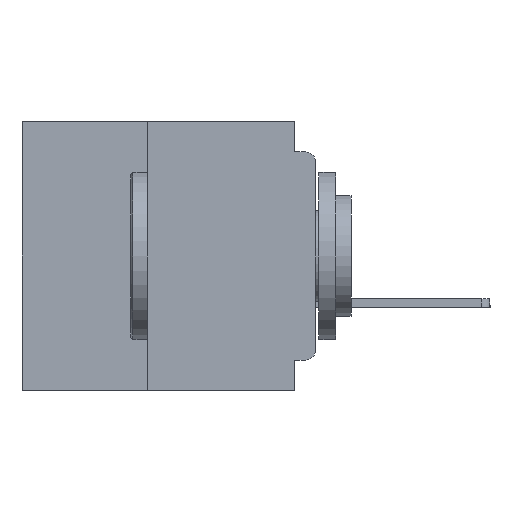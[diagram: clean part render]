
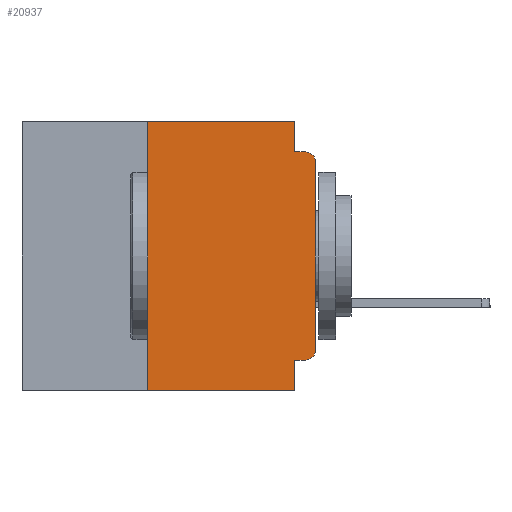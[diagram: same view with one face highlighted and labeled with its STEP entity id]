
A CAD part, left-side view. The second image highlights one B-rep face of the part: STEP entity #20937.
In plain terms, the highlighted planar face has unit normal (-1, 0, 0).
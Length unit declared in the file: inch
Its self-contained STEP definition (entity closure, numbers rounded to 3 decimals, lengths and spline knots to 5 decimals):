
#1321 = LINE ( 'NONE', #22368, #30755 ) ;
#1678 = CARTESIAN_POINT ( 'NONE',  ( 0., 0.25, -0.4 ) ) ;
#2485 = DIRECTION ( 'NONE',  ( 0., 0., -1. ) ) ;
#2578 = VERTEX_POINT ( 'NONE', #18800 ) ;
#4115 = VERTEX_POINT ( 'NONE', #20687 ) ;
#4446 = CARTESIAN_POINT ( 'NONE',  ( 0., 0.031, 0. ) ) ;
#5508 = EDGE_CURVE ( 'NONE', #21175, #4115, #17553, .T. ) ;
#6006 = PLANE ( 'NONE',  #22523 ) ;
#6417 = FACE_OUTER_BOUND ( 'NONE', #26685, .T. ) ;
#6461 = CARTESIAN_POINT ( 'NONE',  ( 0., 0., -0.34 ) ) ;
#6690 = ORIENTED_EDGE ( 'NONE', *, *, #34855, .F. ) ;
#6709 = VECTOR ( 'NONE', #27355, 39.37008 ) ;
#6992 = CIRCLE ( 'NONE', #20363, 0.015 ) ;
#7013 = DIRECTION ( 'NONE',  ( 0., 1., 0. ) ) ;
#7372 = CARTESIAN_POINT ( 'NONE',  ( 0., 0.015, -0.06 ) ) ;
#7402 = EDGE_CURVE ( 'NONE', #34662, #21175, #11601, .T. ) ;
#8612 = VERTEX_POINT ( 'NONE', #4446 ) ;
#8872 = DIRECTION ( 'NONE',  ( 0., 0., -1. ) ) ;
#9820 = CARTESIAN_POINT ( 'NONE',  ( 0., 0.437, -0.4 ) ) ;
#10241 = DIRECTION ( 'NONE',  ( 0., 0., -1. ) ) ;
#10256 = VECTOR ( 'NONE', #13206, 39.37008 ) ;
#10634 = VECTOR ( 'NONE', #2485, 39.37008 ) ;
#10846 = VERTEX_POINT ( 'NONE', #33347 ) ;
#10946 = CARTESIAN_POINT ( 'NONE',  ( 0., 0., -0.045 ) ) ;
#11540 = LINE ( 'NONE', #30866, #10634 ) ;
#11601 = LINE ( 'NONE', #24078, #19231 ) ;
#12197 = CARTESIAN_POINT ( 'NONE',  ( 0., 0.015, -0.355 ) ) ;
#13206 = DIRECTION ( 'NONE',  ( 0., -1., 0. ) ) ;
#13582 = VERTEX_POINT ( 'NONE', #17877 ) ;
#13806 = DIRECTION ( 'NONE',  ( 0., 0., 1. ) ) ;
#13849 = DIRECTION ( 'NONE',  ( 0., -1., 0. ) ) ;
#14216 = ORIENTED_EDGE ( 'NONE', *, *, #5508, .F. ) ;
#14346 = LINE ( 'NONE', #1678, #6709 ) ;
#14812 = ORIENTED_EDGE ( 'NONE', *, *, #19490, .T. ) ;
#15301 = CIRCLE ( 'NONE', #19650, 0.015 ) ;
#16126 = CARTESIAN_POINT ( 'NONE',  ( 0., 0.015, -0.34 ) ) ;
#16238 = ORIENTED_EDGE ( 'NONE', *, *, #29856, .F. ) ;
#16655 = VECTOR ( 'NONE', #26226, 39.37008 ) ;
#17297 = ORIENTED_EDGE ( 'NONE', *, *, #30413, .T. ) ;
#17553 = LINE ( 'NONE', #31826, #16655 ) ;
#17877 = CARTESIAN_POINT ( 'NONE',  ( 0., 0.015, -0.045 ) ) ;
#18475 = DIRECTION ( 'NONE',  ( 0., -1., 0. ) ) ;
#18492 = EDGE_CURVE ( 'NONE', #8612, #2578, #11540, .T. ) ;
#18631 = CARTESIAN_POINT ( 'NONE',  ( 0., 0.031, -0.355 ) ) ;
#18800 = CARTESIAN_POINT ( 'NONE',  ( 0., 0.031, -0.045 ) ) ;
#18992 = DIRECTION ( 'NONE',  ( 0., 0., -1. ) ) ;
#19231 = VECTOR ( 'NONE', #7013, 39.37008 ) ;
#19295 = ORIENTED_EDGE ( 'NONE', *, *, #28532, .T. ) ;
#19490 = EDGE_CURVE ( 'NONE', #34662, #29398, #6992, .T. ) ;
#19650 = AXIS2_PLACEMENT_3D ( 'NONE', #7372, #27225, #10241 ) ;
#20363 = AXIS2_PLACEMENT_3D ( 'NONE', #16126, #35873, #18992 ) ;
#20687 = CARTESIAN_POINT ( 'NONE',  ( 0., 0.031, -0.4 ) ) ;
#20937 = ADVANCED_FACE ( 'NONE', ( #6417 ), #6006, .F. ) ;
#21175 = VERTEX_POINT ( 'NONE', #18631 ) ;
#21303 = VERTEX_POINT ( 'NONE', #33405 ) ;
#22101 = ORIENTED_EDGE ( 'NONE', *, *, #7402, .F. ) ;
#22368 = CARTESIAN_POINT ( 'NONE',  ( 0., 0., 0. ) ) ;
#22523 = AXIS2_PLACEMENT_3D ( 'NONE', #34304, #25891, #8872 ) ;
#24078 = CARTESIAN_POINT ( 'NONE',  ( 0., 0., -0.355 ) ) ;
#25386 = LINE ( 'NONE', #27295, #10256 ) ;
#25891 = DIRECTION ( 'NONE',  ( 1., 0., 0. ) ) ;
#26226 = DIRECTION ( 'NONE',  ( 0., 0., -1. ) ) ;
#26685 = EDGE_LOOP ( 'NONE', ( #19295, #36145, #33596, #32444, #6690, #16238, #17297, #14216, #22101, #14812 ) ) ;
#27225 = DIRECTION ( 'NONE',  ( -1., 0., 0. ) ) ;
#27295 = CARTESIAN_POINT ( 'NONE',  ( 0., 0.437, 0. ) ) ;
#27355 = DIRECTION ( 'NONE',  ( 0., 0., 1. ) ) ;
#28532 = EDGE_CURVE ( 'NONE', #29398, #10846, #1321, .T. ) ;
#29004 = EDGE_CURVE ( 'NONE', #10846, #13582, #15301, .T. ) ;
#29398 = VERTEX_POINT ( 'NONE', #6461 ) ;
#29856 = EDGE_CURVE ( 'NONE', #33048, #21303, #14346, .T. ) ;
#30413 = EDGE_CURVE ( 'NONE', #33048, #4115, #32434, .T. ) ;
#30755 = VECTOR ( 'NONE', #13806, 39.37008 ) ;
#30866 = CARTESIAN_POINT ( 'NONE',  ( 0., 0.031, 0. ) ) ;
#30952 = VECTOR ( 'NONE', #13849, 39.37008 ) ;
#31555 = VECTOR ( 'NONE', #18475, 39.37008 ) ;
#31826 = CARTESIAN_POINT ( 'NONE',  ( 0., 0.031, -0.4 ) ) ;
#32419 = EDGE_CURVE ( 'NONE', #2578, #13582, #32722, .T. ) ;
#32434 = LINE ( 'NONE', #9820, #31555 ) ;
#32444 = ORIENTED_EDGE ( 'NONE', *, *, #18492, .F. ) ;
#32722 = LINE ( 'NONE', #10946, #30952 ) ;
#33012 = CARTESIAN_POINT ( 'NONE',  ( 0., 0.25, -0.4 ) ) ;
#33048 = VERTEX_POINT ( 'NONE', #33012 ) ;
#33347 = CARTESIAN_POINT ( 'NONE',  ( 0., 0., -0.06 ) ) ;
#33405 = CARTESIAN_POINT ( 'NONE',  ( 0., 0.25, 0. ) ) ;
#33596 = ORIENTED_EDGE ( 'NONE', *, *, #32419, .F. ) ;
#34304 = CARTESIAN_POINT ( 'NONE',  ( 0., 0.437, 0. ) ) ;
#34662 = VERTEX_POINT ( 'NONE', #12197 ) ;
#34855 = EDGE_CURVE ( 'NONE', #21303, #8612, #25386, .T. ) ;
#35873 = DIRECTION ( 'NONE',  ( -1., 0., 0. ) ) ;
#36145 = ORIENTED_EDGE ( 'NONE', *, *, #29004, .T. ) ;
